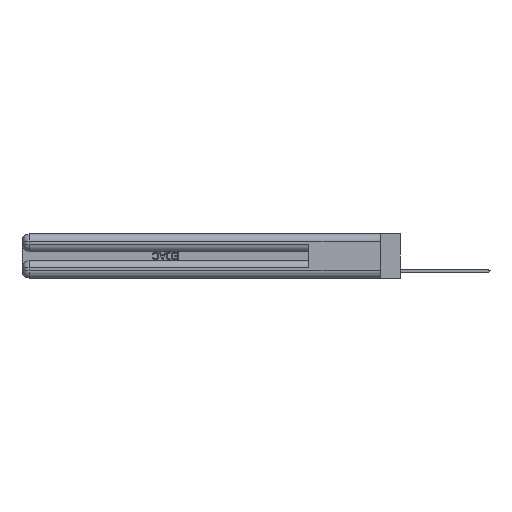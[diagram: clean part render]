
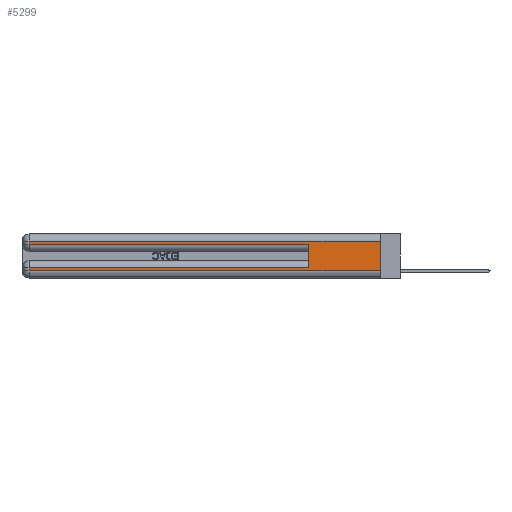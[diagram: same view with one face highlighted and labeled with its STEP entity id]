
A CAD part, left-side view. The second image highlights one B-rep face of the part: STEP entity #5299.
In plain terms, the highlighted planar face has unit normal (-1, 0, 0).
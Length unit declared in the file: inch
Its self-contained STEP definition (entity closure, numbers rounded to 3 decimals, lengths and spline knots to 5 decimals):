
#587 = VERTEX_POINT ( 'NONE', #14559 ) ;
#1000 = ORIENTED_EDGE ( 'NONE', *, *, #15382, .T. ) ;
#1192 = EDGE_LOOP ( 'NONE', ( #26152, #6232, #7238, #14919, #10484, #29445, #1000, #7794 ) ) ;
#1599 = EDGE_CURVE ( 'NONE', #5173, #587, #15734, .T. ) ;
#1725 = CARTESIAN_POINT ( 'NONE',  ( 0., 2.94, 0.285 ) ) ;
#1994 = VECTOR ( 'NONE', #28583, 39.37008 ) ;
#1998 = EDGE_CURVE ( 'NONE', #13003, #22867, #7352, .T. ) ;
#2546 = DIRECTION ( 'NONE',  ( 0., 0., -1. ) ) ;
#4533 = EDGE_CURVE ( 'NONE', #13003, #16914, #11174, .T. ) ;
#5173 = VERTEX_POINT ( 'NONE', #19941 ) ;
#5299 = ADVANCED_FACE ( 'NONE', ( #14034 ), #11332, .F. ) ;
#5935 = DIRECTION ( 'NONE',  ( 0., 0., -1. ) ) ;
#6226 = CARTESIAN_POINT ( 'NONE',  ( 0., 2.94, 0.37 ) ) ;
#6232 = ORIENTED_EDGE ( 'NONE', *, *, #1998, .T. ) ;
#6584 = DIRECTION ( 'NONE',  ( 0., -1., 0. ) ) ;
#7020 = VECTOR ( 'NONE', #9056, 39.37008 ) ;
#7238 = ORIENTED_EDGE ( 'NONE', *, *, #19947, .T. ) ;
#7352 = LINE ( 'NONE', #9315, #10165 ) ;
#7400 = VECTOR ( 'NONE', #15231, 39.37008 ) ;
#7633 = VERTEX_POINT ( 'NONE', #12312 ) ;
#7794 = ORIENTED_EDGE ( 'NONE', *, *, #27882, .T. ) ;
#9056 = DIRECTION ( 'NONE',  ( 0., 0., -1. ) ) ;
#9315 = CARTESIAN_POINT ( 'NONE',  ( 0., 0., 0.31 ) ) ;
#9971 = LINE ( 'NONE', #23872, #7400 ) ;
#10165 = VECTOR ( 'NONE', #27752, 39.37008 ) ;
#10484 = ORIENTED_EDGE ( 'NONE', *, *, #10731, .F. ) ;
#10731 = EDGE_CURVE ( 'NONE', #5173, #28042, #13011, .T. ) ;
#11113 = CARTESIAN_POINT ( 'NONE',  ( 0., 0., 0.06 ) ) ;
#11174 = LINE ( 'NONE', #29757, #7020 ) ;
#11332 = PLANE ( 'NONE',  #13795 ) ;
#12312 = CARTESIAN_POINT ( 'NONE',  ( 0., 2.94, 0.06 ) ) ;
#12334 = CARTESIAN_POINT ( 'NONE',  ( 0., 0., 0.31 ) ) ;
#12864 = CARTESIAN_POINT ( 'NONE',  ( 0., 0.6, 0.145 ) ) ;
#13003 = VERTEX_POINT ( 'NONE', #12334 ) ;
#13011 = LINE ( 'NONE', #12864, #19237 ) ;
#13795 = AXIS2_PLACEMENT_3D ( 'NONE', #16156, #27796, #2546 ) ;
#13884 = EDGE_CURVE ( 'NONE', #15890, #28042, #26451, .T. ) ;
#14034 = FACE_OUTER_BOUND ( 'NONE', #1192, .T. ) ;
#14234 = CARTESIAN_POINT ( 'NONE',  ( 0., 0., 0.06 ) ) ;
#14559 = CARTESIAN_POINT ( 'NONE',  ( 0., 2.94, 0.085 ) ) ;
#14919 = ORIENTED_EDGE ( 'NONE', *, *, #13884, .T. ) ;
#15231 = DIRECTION ( 'NONE',  ( 0., 0., -1. ) ) ;
#15382 = EDGE_CURVE ( 'NONE', #587, #7633, #9971, .T. ) ;
#15734 = LINE ( 'NONE', #20551, #15844 ) ;
#15844 = VECTOR ( 'NONE', #29791, 39.37008 ) ;
#15890 = VERTEX_POINT ( 'NONE', #1725 ) ;
#16156 = CARTESIAN_POINT ( 'NONE',  ( 0., 0., 0.37 ) ) ;
#16545 = CARTESIAN_POINT ( 'NONE',  ( 0., 2.94, 0.31 ) ) ;
#16914 = VERTEX_POINT ( 'NONE', #14234 ) ;
#18641 = VECTOR ( 'NONE', #6584, 39.37008 ) ;
#19237 = VECTOR ( 'NONE', #22229, 39.37008 ) ;
#19941 = CARTESIAN_POINT ( 'NONE',  ( 0., 0.6, 0.085 ) ) ;
#19947 = EDGE_CURVE ( 'NONE', #22867, #15890, #28611, .T. ) ;
#20551 = CARTESIAN_POINT ( 'NONE',  ( 0., 0., 0.085 ) ) ;
#22229 = DIRECTION ( 'NONE',  ( 0., 0., 1. ) ) ;
#22296 = LINE ( 'NONE', #11113, #18641 ) ;
#22867 = VERTEX_POINT ( 'NONE', #16545 ) ;
#23872 = CARTESIAN_POINT ( 'NONE',  ( 0., 2.94, 0.37 ) ) ;
#24657 = VECTOR ( 'NONE', #5935, 39.37008 ) ;
#25762 = CARTESIAN_POINT ( 'NONE',  ( 0., 0.6, 0.285 ) ) ;
#26152 = ORIENTED_EDGE ( 'NONE', *, *, #4533, .F. ) ;
#26153 = CARTESIAN_POINT ( 'NONE',  ( 0., 0., 0.285 ) ) ;
#26451 = LINE ( 'NONE', #26153, #1994 ) ;
#27752 = DIRECTION ( 'NONE',  ( 0., 1., 0. ) ) ;
#27796 = DIRECTION ( 'NONE',  ( 1., 0., 0. ) ) ;
#27882 = EDGE_CURVE ( 'NONE', #7633, #16914, #22296, .T. ) ;
#28042 = VERTEX_POINT ( 'NONE', #25762 ) ;
#28583 = DIRECTION ( 'NONE',  ( 0., -1., 0. ) ) ;
#28611 = LINE ( 'NONE', #6226, #24657 ) ;
#29445 = ORIENTED_EDGE ( 'NONE', *, *, #1599, .T. ) ;
#29757 = CARTESIAN_POINT ( 'NONE',  ( 0., 0., 0.37 ) ) ;
#29791 = DIRECTION ( 'NONE',  ( 0., 1., 0. ) ) ;
